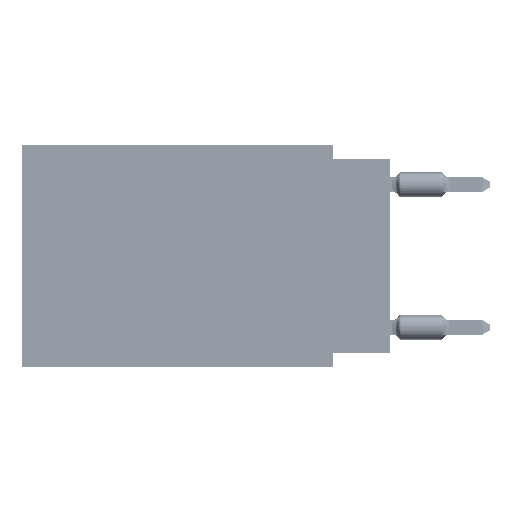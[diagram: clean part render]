
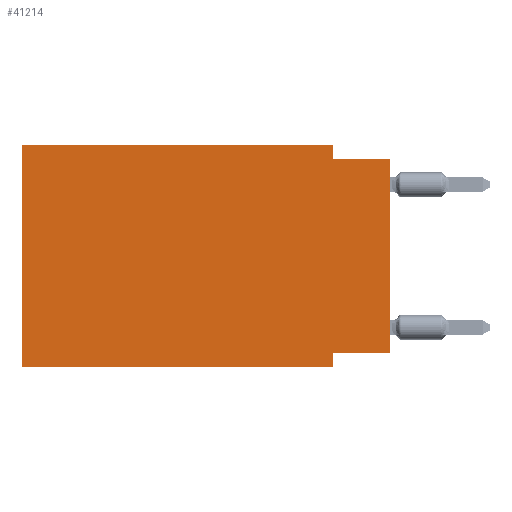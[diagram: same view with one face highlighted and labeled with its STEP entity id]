
A CAD part, left-side view. The second image highlights one B-rep face of the part: STEP entity #41214.
In plain terms, the highlighted planar face has unit normal (-1, 0, 0).
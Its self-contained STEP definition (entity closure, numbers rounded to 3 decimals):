
#253 = EDGE_CURVE ( 'NONE', #47393, #57086, #65524, .T. ) ;
#1682 = CARTESIAN_POINT ( 'NONE',  ( 0., 0., 0. ) ) ;
#3233 = DIRECTION ( 'NONE',  ( 0., -1., 0. ) ) ;
#5306 = CARTESIAN_POINT ( 'NONE',  ( 0., 2.54, -0.635 ) ) ;
#9330 = CARTESIAN_POINT ( 'NONE',  ( 0., 16.383, 0. ) ) ;
#9884 = VERTEX_POINT ( 'NONE', #67924 ) ;
#12472 = CARTESIAN_POINT ( 'NONE',  ( 0., 0., -0.635 ) ) ;
#13839 = EDGE_CURVE ( 'NONE', #9884, #24822, #72383, .T. ) ;
#14011 = DIRECTION ( 'NONE',  ( 0., -1., 0. ) ) ;
#14217 = ORIENTED_EDGE ( 'NONE', *, *, #46474, .F. ) ;
#15125 = CARTESIAN_POINT ( 'NONE',  ( 0., 2.54, 0. ) ) ;
#16091 = ORIENTED_EDGE ( 'NONE', *, *, #74380, .F. ) ;
#18408 = DIRECTION ( 'NONE',  ( 0., 0., -1. ) ) ;
#19850 = VECTOR ( 'NONE', #78563, 1000. ) ;
#23425 = LINE ( 'NONE', #74641, #62042 ) ;
#24336 = VECTOR ( 'NONE', #67265, 1000. ) ;
#24822 = VERTEX_POINT ( 'NONE', #35067 ) ;
#25082 = DIRECTION ( 'NONE',  ( 0., -1., 0. ) ) ;
#28494 = VERTEX_POINT ( 'NONE', #82043 ) ;
#28782 = VERTEX_POINT ( 'NONE', #9330 ) ;
#30171 = CARTESIAN_POINT ( 'NONE',  ( 0., 0., -9.271 ) ) ;
#30491 = VECTOR ( 'NONE', #18408, 1000. ) ;
#30989 = ORIENTED_EDGE ( 'NONE', *, *, #82013, .F. ) ;
#31464 = PLANE ( 'NONE',  #44700 ) ;
#35067 = CARTESIAN_POINT ( 'NONE',  ( 0., 2.54, -9.906 ) ) ;
#35241 = ORIENTED_EDGE ( 'NONE', *, *, #39162, .F. ) ;
#36601 = EDGE_LOOP ( 'NONE', ( #37429, #14217, #16091, #45866, #43079, #45429, #35241, #30989 ) ) ;
#37429 = ORIENTED_EDGE ( 'NONE', *, *, #253, .T. ) ;
#38118 = DIRECTION ( 'NONE',  ( 0., 1., 0. ) ) ;
#39162 = EDGE_CURVE ( 'NONE', #28494, #24822, #66026, .T. ) ;
#40400 = VERTEX_POINT ( 'NONE', #5306 ) ;
#41214 = ADVANCED_FACE ( 'NONE', ( #57894 ), #31464, .F. ) ;
#41854 = CARTESIAN_POINT ( 'NONE',  ( 0., 16.383, 0. ) ) ;
#42274 = LINE ( 'NONE', #41854, #45416 ) ;
#42502 = VECTOR ( 'NONE', #25082, 1000. ) ;
#43079 = ORIENTED_EDGE ( 'NONE', *, *, #64864, .F. ) ;
#44700 = AXIS2_PLACEMENT_3D ( 'NONE', #63772, #50374, #70894 ) ;
#45416 = VECTOR ( 'NONE', #3233, 1000. ) ;
#45429 = ORIENTED_EDGE ( 'NONE', *, *, #13839, .T. ) ;
#45866 = ORIENTED_EDGE ( 'NONE', *, *, #54291, .F. ) ;
#45917 = CARTESIAN_POINT ( 'NONE',  ( 0., 16.383, -9.906 ) ) ;
#46474 = EDGE_CURVE ( 'NONE', #40400, #57086, #58643, .T. ) ;
#47393 = VERTEX_POINT ( 'NONE', #73431 ) ;
#50312 = LINE ( 'NONE', #30171, #71280 ) ;
#50374 = DIRECTION ( 'NONE',  ( 1., 0., 0. ) ) ;
#53455 = CARTESIAN_POINT ( 'NONE',  ( 0., 2.54, -9.906 ) ) ;
#54291 = EDGE_CURVE ( 'NONE', #28782, #77003, #42274, .T. ) ;
#57086 = VERTEX_POINT ( 'NONE', #61216 ) ;
#57894 = FACE_OUTER_BOUND ( 'NONE', #36601, .T. ) ;
#58643 = LINE ( 'NONE', #12472, #42502 ) ;
#60384 = VECTOR ( 'NONE', #14011, 1000. ) ;
#61216 = CARTESIAN_POINT ( 'NONE',  ( 0., 0., -0.635 ) ) ;
#62042 = VECTOR ( 'NONE', #81367, 1000. ) ;
#63772 = CARTESIAN_POINT ( 'NONE',  ( 0., 16.383, 0. ) ) ;
#64864 = EDGE_CURVE ( 'NONE', #9884, #28782, #23425, .T. ) ;
#65524 = LINE ( 'NONE', #1682, #19850 ) ;
#66026 = LINE ( 'NONE', #53455, #24336 ) ;
#67265 = DIRECTION ( 'NONE',  ( 0., 0., -1. ) ) ;
#67924 = CARTESIAN_POINT ( 'NONE',  ( 0., 16.383, -9.906 ) ) ;
#69631 = LINE ( 'NONE', #75942, #30491 ) ;
#70894 = DIRECTION ( 'NONE',  ( 0., 0., -1. ) ) ;
#71280 = VECTOR ( 'NONE', #38118, 1000. ) ;
#72383 = LINE ( 'NONE', #45917, #60384 ) ;
#73431 = CARTESIAN_POINT ( 'NONE',  ( 0., 0., -9.271 ) ) ;
#74380 = EDGE_CURVE ( 'NONE', #77003, #40400, #69631, .T. ) ;
#74641 = CARTESIAN_POINT ( 'NONE',  ( 0., 16.383, 0. ) ) ;
#75942 = CARTESIAN_POINT ( 'NONE',  ( 0., 2.54, 0. ) ) ;
#77003 = VERTEX_POINT ( 'NONE', #15125 ) ;
#78563 = DIRECTION ( 'NONE',  ( 0., 0., 1. ) ) ;
#81367 = DIRECTION ( 'NONE',  ( 0., 0., 1. ) ) ;
#82013 = EDGE_CURVE ( 'NONE', #47393, #28494, #50312, .T. ) ;
#82043 = CARTESIAN_POINT ( 'NONE',  ( 0., 2.54, -9.271 ) ) ;
